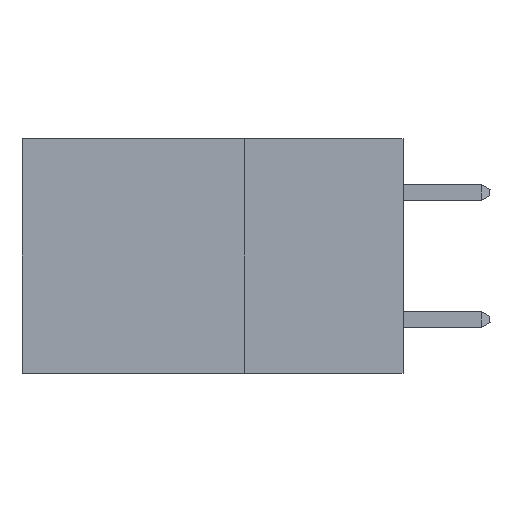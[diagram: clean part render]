
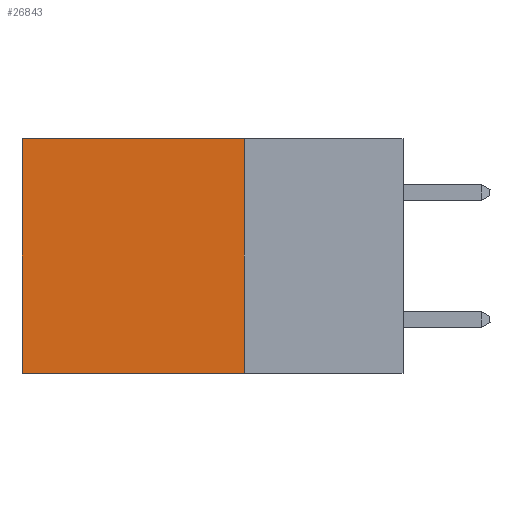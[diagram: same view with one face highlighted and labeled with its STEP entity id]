
A CAD part, left-side view. The second image highlights one B-rep face of the part: STEP entity #26843.
In plain terms, the highlighted planar face has unit normal (-1, 0, 0).
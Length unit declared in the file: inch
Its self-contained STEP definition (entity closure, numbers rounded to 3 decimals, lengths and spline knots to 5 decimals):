
#2276 = ORIENTED_EDGE ( 'NONE', *, *, #39368, .F. ) ;
#3533 = PLANE ( 'NONE',  #11134 ) ;
#3972 = CARTESIAN_POINT ( 'NONE',  ( 0.2875, 0.6, -0.37 ) ) ;
#4771 = EDGE_CURVE ( 'NONE', #6781, #19195, #28253, .T. ) ;
#5085 = ORIENTED_EDGE ( 'NONE', *, *, #37113, .F. ) ;
#5733 = CARTESIAN_POINT ( 'NONE',  ( 0.2875, 0.6, 0. ) ) ;
#6781 = VERTEX_POINT ( 'NONE', #25413 ) ;
#7111 = VECTOR ( 'NONE', #16376, 39.37008 ) ;
#8460 = ORIENTED_EDGE ( 'NONE', *, *, #29221, .T. ) ;
#8474 = VECTOR ( 'NONE', #19790, 39.37008 ) ;
#9008 = LINE ( 'NONE', #38978, #8474 ) ;
#9622 = CARTESIAN_POINT ( 'NONE',  ( 0.2875, 0.25, 0. ) ) ;
#11134 = AXIS2_PLACEMENT_3D ( 'NONE', #16668, #25940, #35583 ) ;
#13184 = CARTESIAN_POINT ( 'NONE',  ( 0.2875, 0.25, -0.37 ) ) ;
#13655 = VECTOR ( 'NONE', #28372, 39.37008 ) ;
#15209 = CARTESIAN_POINT ( 'NONE',  ( 0.2875, 0.25, 0. ) ) ;
#16376 = DIRECTION ( 'NONE',  ( 0., 1., 0. ) ) ;
#16668 = CARTESIAN_POINT ( 'NONE',  ( 0.2875, 0.25, 0. ) ) ;
#19195 = VERTEX_POINT ( 'NONE', #3972 ) ;
#19790 = DIRECTION ( 'NONE',  ( 0., 1., 0. ) ) ;
#25413 = CARTESIAN_POINT ( 'NONE',  ( 0.2875, 0.6, 0. ) ) ;
#25940 = DIRECTION ( 'NONE',  ( 1., 0., 0. ) ) ;
#26623 = VERTEX_POINT ( 'NONE', #9622 ) ;
#26701 = FACE_OUTER_BOUND ( 'NONE', #27806, .T. ) ;
#26726 = VECTOR ( 'NONE', #34284, 39.37008 ) ;
#26843 = ADVANCED_FACE ( 'NONE', ( #26701 ), #3533, .F. ) ;
#27806 = EDGE_LOOP ( 'NONE', ( #34738, #5085, #2276, #8460 ) ) ;
#28253 = LINE ( 'NONE', #5733, #26726 ) ;
#28372 = DIRECTION ( 'NONE',  ( 0., 0., -1. ) ) ;
#29221 = EDGE_CURVE ( 'NONE', #26623, #6781, #9008, .T. ) ;
#30782 = VERTEX_POINT ( 'NONE', #34800 ) ;
#33201 = LINE ( 'NONE', #15209, #13655 ) ;
#34284 = DIRECTION ( 'NONE',  ( 0., 0., -1. ) ) ;
#34738 = ORIENTED_EDGE ( 'NONE', *, *, #4771, .T. ) ;
#34800 = CARTESIAN_POINT ( 'NONE',  ( 0.2875, 0.25, -0.37 ) ) ;
#35583 = DIRECTION ( 'NONE',  ( 0., 0., -1. ) ) ;
#37113 = EDGE_CURVE ( 'NONE', #30782, #19195, #40640, .T. ) ;
#38978 = CARTESIAN_POINT ( 'NONE',  ( 0.2875, 0.25, 0. ) ) ;
#39368 = EDGE_CURVE ( 'NONE', #26623, #30782, #33201, .T. ) ;
#40640 = LINE ( 'NONE', #13184, #7111 ) ;
